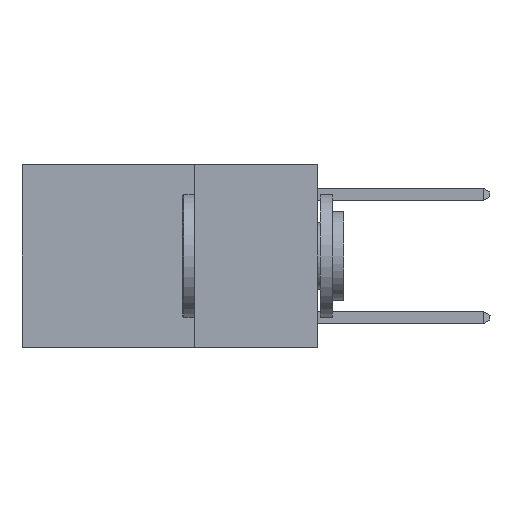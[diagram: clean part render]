
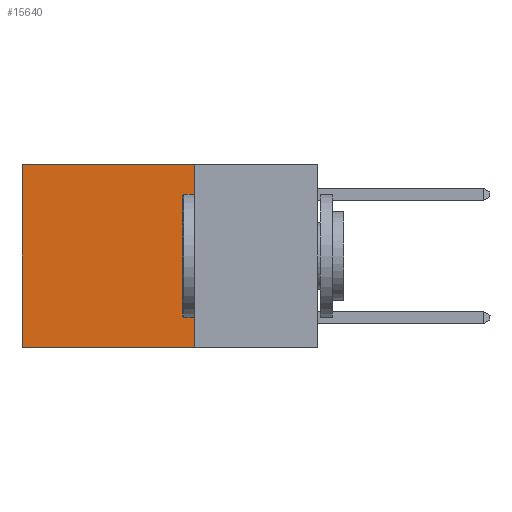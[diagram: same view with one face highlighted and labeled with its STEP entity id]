
A CAD part, left-side view. The second image highlights one B-rep face of the part: STEP entity #15640.
In plain terms, the highlighted planar face has unit normal (-1, 0, 0).
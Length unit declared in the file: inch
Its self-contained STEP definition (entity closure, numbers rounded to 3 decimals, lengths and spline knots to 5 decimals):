
#247 = VERTEX_POINT ( 'NONE', #8792 ) ;
#526 = DIRECTION ( 'NONE',  ( 0., 0., -1. ) ) ;
#1083 = FACE_OUTER_BOUND ( 'NONE', #25980, .T. ) ;
#1312 = DIRECTION ( 'NONE',  ( 0., 0., -1. ) ) ;
#2442 = VECTOR ( 'NONE', #1312, 39.37008 ) ;
#4053 = VECTOR ( 'NONE', #5333, 39.37008 ) ;
#4535 = LINE ( 'NONE', #26389, #2442 ) ;
#5333 = DIRECTION ( 'NONE',  ( 0., 1., 0. ) ) ;
#5390 = PLANE ( 'NONE',  #7151 ) ;
#5428 = CARTESIAN_POINT ( 'NONE',  ( 0.2625, 0.6, 0. ) ) ;
#6161 = ORIENTED_EDGE ( 'NONE', *, *, #13617, .F. ) ;
#6269 = VERTEX_POINT ( 'NONE', #5428 ) ;
#6403 = CARTESIAN_POINT ( 'NONE',  ( 0.2625, 0.25, 0. ) ) ;
#6530 = DIRECTION ( 'NONE',  ( 0., 0., -1. ) ) ;
#7151 = AXIS2_PLACEMENT_3D ( 'NONE', #17629, #11089, #526 ) ;
#8503 = EDGE_CURVE ( 'NONE', #25380, #247, #20434, .T. ) ;
#8792 = CARTESIAN_POINT ( 'NONE',  ( 0.2625, 0.6, -0.37 ) ) ;
#9326 = EDGE_CURVE ( 'NONE', #6269, #247, #4535, .T. ) ;
#11089 = DIRECTION ( 'NONE',  ( 1., 0., 0. ) ) ;
#13617 = EDGE_CURVE ( 'NONE', #20962, #25380, #21290, .T. ) ;
#15496 = VECTOR ( 'NONE', #6530, 39.37008 ) ;
#15640 = ADVANCED_FACE ( 'NONE', ( #1083 ), #5390, .F. ) ;
#16541 = DIRECTION ( 'NONE',  ( 0., 1., 0. ) ) ;
#17463 = EDGE_CURVE ( 'NONE', #20962, #6269, #26220, .T. ) ;
#17629 = CARTESIAN_POINT ( 'NONE',  ( 0.2625, 0.25, 0. ) ) ;
#17762 = CARTESIAN_POINT ( 'NONE',  ( 0.2625, 0.25, -0.37 ) ) ;
#18350 = CARTESIAN_POINT ( 'NONE',  ( 0.2625, 0.25, -0.37 ) ) ;
#19945 = CARTESIAN_POINT ( 'NONE',  ( 0.2625, 0.25, 0. ) ) ;
#20300 = ORIENTED_EDGE ( 'NONE', *, *, #8503, .F. ) ;
#20434 = LINE ( 'NONE', #18350, #26439 ) ;
#20962 = VERTEX_POINT ( 'NONE', #21161 ) ;
#21161 = CARTESIAN_POINT ( 'NONE',  ( 0.2625, 0.25, 0. ) ) ;
#21290 = LINE ( 'NONE', #6403, #15496 ) ;
#23776 = ORIENTED_EDGE ( 'NONE', *, *, #9326, .T. ) ;
#25242 = ORIENTED_EDGE ( 'NONE', *, *, #17463, .T. ) ;
#25380 = VERTEX_POINT ( 'NONE', #17762 ) ;
#25980 = EDGE_LOOP ( 'NONE', ( #23776, #20300, #6161, #25242 ) ) ;
#26220 = LINE ( 'NONE', #19945, #4053 ) ;
#26389 = CARTESIAN_POINT ( 'NONE',  ( 0.2625, 0.6, 0. ) ) ;
#26439 = VECTOR ( 'NONE', #16541, 39.37008 ) ;
